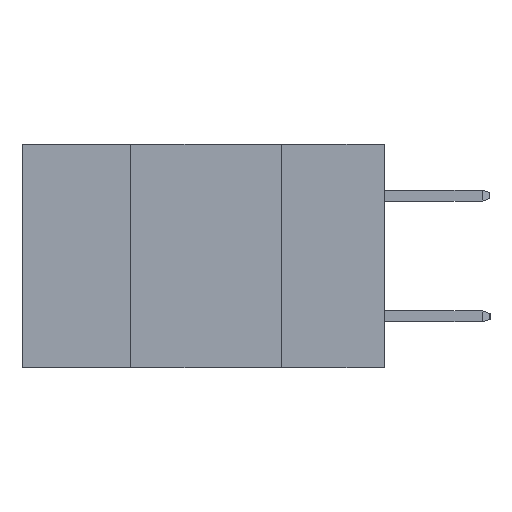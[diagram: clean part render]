
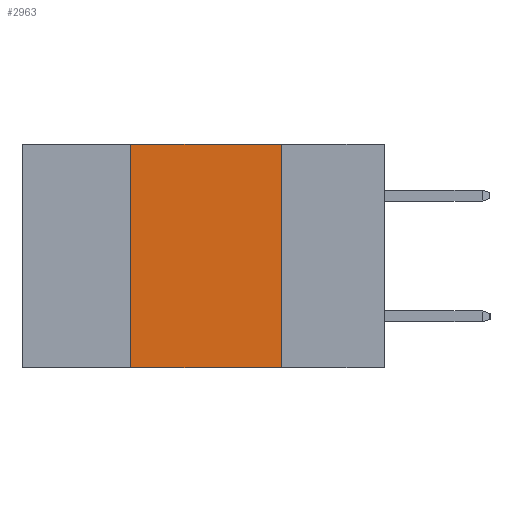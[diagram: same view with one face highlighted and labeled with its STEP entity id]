
A CAD part, left-side view. The second image highlights one B-rep face of the part: STEP entity #2963.
In plain terms, the highlighted planar face has unit normal (-1, 0, 0).
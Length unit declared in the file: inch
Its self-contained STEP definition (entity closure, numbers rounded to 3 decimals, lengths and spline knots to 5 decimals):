
#658 = VERTEX_POINT ( 'NONE', #8511 ) ;
#930 = ORIENTED_EDGE ( 'NONE', *, *, #4973, .F. ) ;
#1519 = DIRECTION ( 'NONE',  ( 0., 0., -1. ) ) ;
#1625 = VERTEX_POINT ( 'NONE', #3486 ) ;
#1667 = DIRECTION ( 'NONE',  ( 1., 0., 0. ) ) ;
#1756 = ORIENTED_EDGE ( 'NONE', *, *, #6677, .F. ) ;
#2112 = ORIENTED_EDGE ( 'NONE', *, *, #8291, .T. ) ;
#2146 = DIRECTION ( 'NONE',  ( 0., 0., -1. ) ) ;
#2155 = PLANE ( 'NONE',  #3974 ) ;
#2503 = VECTOR ( 'NONE', #2146, 39.37008 ) ;
#2963 = ADVANCED_FACE ( 'NONE', ( #8670 ), #2155, .F. ) ;
#3077 = VECTOR ( 'NONE', #3476, 39.37008 ) ;
#3223 = CARTESIAN_POINT ( 'NONE',  ( 0., 0.42, -0.37 ) ) ;
#3476 = DIRECTION ( 'NONE',  ( 0., -1., 0. ) ) ;
#3486 = CARTESIAN_POINT ( 'NONE',  ( 0., 0.42, 0. ) ) ;
#3544 = CARTESIAN_POINT ( 'NONE',  ( 0., 0.17, 0. ) ) ;
#3662 = CARTESIAN_POINT ( 'NONE',  ( 0., 0.6, 0. ) ) ;
#3974 = AXIS2_PLACEMENT_3D ( 'NONE', #3662, #1667, #1519 ) ;
#4396 = VERTEX_POINT ( 'NONE', #3544 ) ;
#4973 = EDGE_CURVE ( 'NONE', #1625, #4396, #9468, .T. ) ;
#5181 = ORIENTED_EDGE ( 'NONE', *, *, #10049, .F. ) ;
#5720 = CARTESIAN_POINT ( 'NONE',  ( 0., 0.6, 0. ) ) ;
#5725 = DIRECTION ( 'NONE',  ( 0., -1., 0. ) ) ;
#6484 = CARTESIAN_POINT ( 'NONE',  ( 0., 0.17, -0.37 ) ) ;
#6677 = EDGE_CURVE ( 'NONE', #8121, #1625, #8270, .T. ) ;
#7050 = LINE ( 'NONE', #6484, #2503 ) ;
#7369 = VECTOR ( 'NONE', #5725, 39.37008 ) ;
#7845 = EDGE_LOOP ( 'NONE', ( #5181, #930, #1756, #2112 ) ) ;
#7847 = LINE ( 'NONE', #9311, #3077 ) ;
#8121 = VERTEX_POINT ( 'NONE', #10635 ) ;
#8270 = LINE ( 'NONE', #3223, #9870 ) ;
#8278 = DIRECTION ( 'NONE',  ( 0., 0., 1. ) ) ;
#8291 = EDGE_CURVE ( 'NONE', #8121, #658, #7847, .T. ) ;
#8511 = CARTESIAN_POINT ( 'NONE',  ( 0., 0.17, -0.37 ) ) ;
#8670 = FACE_OUTER_BOUND ( 'NONE', #7845, .T. ) ;
#9311 = CARTESIAN_POINT ( 'NONE',  ( 0., 0.6, -0.37 ) ) ;
#9468 = LINE ( 'NONE', #5720, #7369 ) ;
#9870 = VECTOR ( 'NONE', #8278, 39.37008 ) ;
#10049 = EDGE_CURVE ( 'NONE', #4396, #658, #7050, .T. ) ;
#10635 = CARTESIAN_POINT ( 'NONE',  ( 0., 0.42, -0.37 ) ) ;
